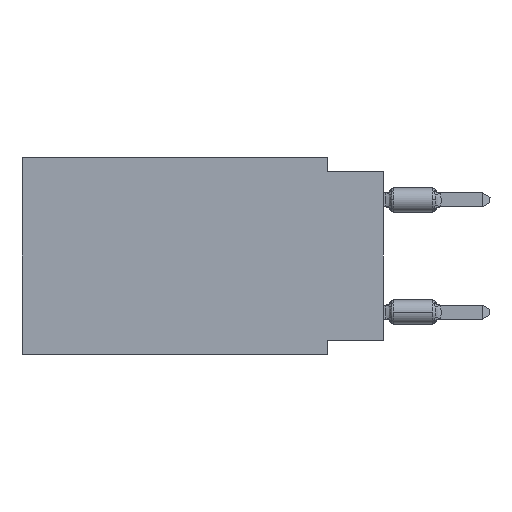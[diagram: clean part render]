
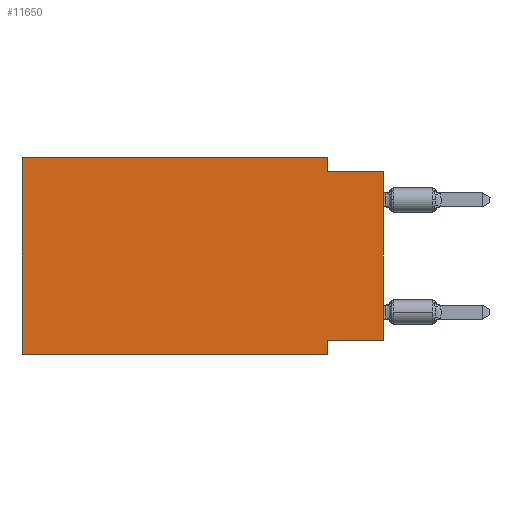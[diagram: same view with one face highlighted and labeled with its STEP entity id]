
A CAD part, left-side view. The second image highlights one B-rep face of the part: STEP entity #11650.
In plain terms, the highlighted planar face has unit normal (-1, 0, 0).
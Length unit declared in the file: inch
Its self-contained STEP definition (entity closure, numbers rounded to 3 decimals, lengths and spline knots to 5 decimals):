
#552 = ORIENTED_EDGE ( 'NONE', *, *, #47139, .F. ) ;
#1874 = VERTEX_POINT ( 'NONE', #1923 ) ;
#1923 = CARTESIAN_POINT ( 'NONE',  ( 0., 0.1, -0.35 ) ) ;
#2710 = LINE ( 'NONE', #43100, #34154 ) ;
#2818 = LINE ( 'NONE', #7476, #35212 ) ;
#3576 = LINE ( 'NONE', #13228, #21688 ) ;
#4114 = LINE ( 'NONE', #29633, #12063 ) ;
#4799 = VERTEX_POINT ( 'NONE', #24293 ) ;
#6546 = EDGE_CURVE ( 'NONE', #27103, #4799, #2710, .T. ) ;
#6887 = ORIENTED_EDGE ( 'NONE', *, *, #23911, .F. ) ;
#7476 = CARTESIAN_POINT ( 'NONE',  ( 0., 0.1, 0. ) ) ;
#7509 = ORIENTED_EDGE ( 'NONE', *, *, #41079, .F. ) ;
#7882 = VERTEX_POINT ( 'NONE', #48876 ) ;
#8357 = DIRECTION ( 'NONE',  ( 0., 0., -1. ) ) ;
#8902 = DIRECTION ( 'NONE',  ( 0., 0., 1. ) ) ;
#10466 = VERTEX_POINT ( 'NONE', #17543 ) ;
#10482 = ORIENTED_EDGE ( 'NONE', *, *, #28085, .F. ) ;
#11650 = ADVANCED_FACE ( 'NONE', ( #49065 ), #13642, .F. ) ;
#12063 = VECTOR ( 'NONE', #47509, 39.37008 ) ;
#13228 = CARTESIAN_POINT ( 'NONE',  ( 0., 0.1, -0.35 ) ) ;
#13278 = DIRECTION ( 'NONE',  ( 0., -1., 0. ) ) ;
#13600 = CARTESIAN_POINT ( 'NONE',  ( 0., 0.645, 0. ) ) ;
#13642 = PLANE ( 'NONE',  #56521 ) ;
#14669 = ORIENTED_EDGE ( 'NONE', *, *, #26061, .F. ) ;
#17543 = CARTESIAN_POINT ( 'NONE',  ( 0., 0.1, 0. ) ) ;
#17580 = EDGE_CURVE ( 'NONE', #37370, #4799, #33417, .T. ) ;
#17672 = LINE ( 'NONE', #44300, #20720 ) ;
#20720 = VECTOR ( 'NONE', #13278, 39.37008 ) ;
#21688 = VECTOR ( 'NONE', #39859, 39.37008 ) ;
#23911 = EDGE_CURVE ( 'NONE', #10466, #37370, #2818, .T. ) ;
#24293 = CARTESIAN_POINT ( 'NONE',  ( 0., 0., -0.025 ) ) ;
#25525 = DIRECTION ( 'NONE',  ( 0., 0., 1. ) ) ;
#26061 = EDGE_CURVE ( 'NONE', #50979, #7882, #52552, .T. ) ;
#27103 = VERTEX_POINT ( 'NONE', #46150 ) ;
#28085 = EDGE_CURVE ( 'NONE', #7882, #10466, #4114, .T. ) ;
#29633 = CARTESIAN_POINT ( 'NONE',  ( 0., 0.645, 0. ) ) ;
#30911 = CARTESIAN_POINT ( 'NONE',  ( 0., 0.645, 0. ) ) ;
#33381 = VECTOR ( 'NONE', #8902, 39.37008 ) ;
#33417 = LINE ( 'NONE', #54526, #37248 ) ;
#33484 = CARTESIAN_POINT ( 'NONE',  ( 0., 0.645, -0.35 ) ) ;
#34154 = VECTOR ( 'NONE', #25525, 39.37008 ) ;
#34163 = CARTESIAN_POINT ( 'NONE',  ( 0., 0., -0.325 ) ) ;
#34260 = ORIENTED_EDGE ( 'NONE', *, *, #40627, .T. ) ;
#34746 = DIRECTION ( 'NONE',  ( 0., 1., 0. ) ) ;
#35212 = VECTOR ( 'NONE', #8357, 39.37008 ) ;
#35871 = DIRECTION ( 'NONE',  ( 1., 0., 0. ) ) ;
#36414 = VERTEX_POINT ( 'NONE', #44703 ) ;
#36668 = DIRECTION ( 'NONE',  ( 0., -1., 0. ) ) ;
#36674 = CARTESIAN_POINT ( 'NONE',  ( 0., 0.1, -0.025 ) ) ;
#37248 = VECTOR ( 'NONE', #36668, 39.37008 ) ;
#37370 = VERTEX_POINT ( 'NONE', #36674 ) ;
#39859 = DIRECTION ( 'NONE',  ( 0., 0., -1. ) ) ;
#40045 = ORIENTED_EDGE ( 'NONE', *, *, #17580, .F. ) ;
#40627 = EDGE_CURVE ( 'NONE', #50979, #1874, #17672, .T. ) ;
#41079 = EDGE_CURVE ( 'NONE', #36414, #1874, #3576, .T. ) ;
#43100 = CARTESIAN_POINT ( 'NONE',  ( 0., 0., 0. ) ) ;
#44300 = CARTESIAN_POINT ( 'NONE',  ( 0., 0.645, -0.35 ) ) ;
#44703 = CARTESIAN_POINT ( 'NONE',  ( 0., 0.1, -0.325 ) ) ;
#46150 = CARTESIAN_POINT ( 'NONE',  ( 0., 0., -0.325 ) ) ;
#47139 = EDGE_CURVE ( 'NONE', #27103, #36414, #57576, .T. ) ;
#47499 = VECTOR ( 'NONE', #34746, 39.37008 ) ;
#47509 = DIRECTION ( 'NONE',  ( 0., -1., 0. ) ) ;
#48786 = DIRECTION ( 'NONE',  ( 0., 0., -1. ) ) ;
#48876 = CARTESIAN_POINT ( 'NONE',  ( 0., 0.645, 0. ) ) ;
#49065 = FACE_OUTER_BOUND ( 'NONE', #53794, .T. ) ;
#50979 = VERTEX_POINT ( 'NONE', #33484 ) ;
#52552 = LINE ( 'NONE', #13600, #33381 ) ;
#53794 = EDGE_LOOP ( 'NONE', ( #56784, #40045, #6887, #10482, #14669, #34260, #7509, #552 ) ) ;
#54526 = CARTESIAN_POINT ( 'NONE',  ( 0., 0., -0.025 ) ) ;
#56521 = AXIS2_PLACEMENT_3D ( 'NONE', #30911, #35871, #48786 ) ;
#56784 = ORIENTED_EDGE ( 'NONE', *, *, #6546, .T. ) ;
#57576 = LINE ( 'NONE', #34163, #47499 ) ;
